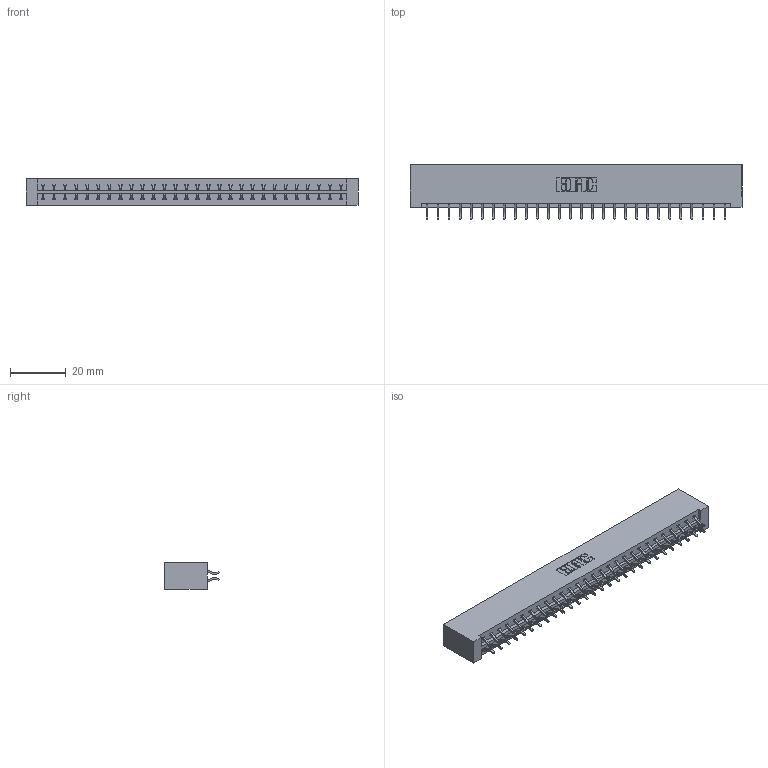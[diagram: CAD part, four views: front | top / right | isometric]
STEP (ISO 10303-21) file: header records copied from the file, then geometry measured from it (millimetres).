
FILE_DESCRIPTION (( 'STEP AP203' ), '1' );
FILE_NAME ('833-056-556-201.STEP', '2020-06-04T23:15:57', ( '' ), ( '' ), 'SwSTEP 2.0', 'SolidWorks 2020', '' );
FILE_SCHEMA (( 'CONFIG_CONTROL_DESIGN' ));
Length unit declared in the file: inch
Products named in the file (3): 345-292-001_556 Tail; 833 Part_Lugless; 833-056-556-201
Assembly tree (57 placements, depth 2):
  833-056-556-201
    833 Part_Lugless
    345-292-001_556 Tail  x56
Bounding box: 119.2 x 19.57 x 9.4 mm (x, y, z)
Volume: 12669 mm3; surface area: 14796.5 mm2
Topology: 57 solids, 57 shells, 3354 faces, 9975 edges, 6574 vertices
Faces by surface type: plane 2306, cylinder 1048
Entity records: 19767 total; most frequent: CARTESIAN_POINT 3306, ORIENTED_EDGE 3230, DIRECTION 2831, EDGE_CURVE 1615, LINE 1487, VECTOR 1487, VERTEX_POINT 1074, AXIS2_PLACEMENT_3D 672
